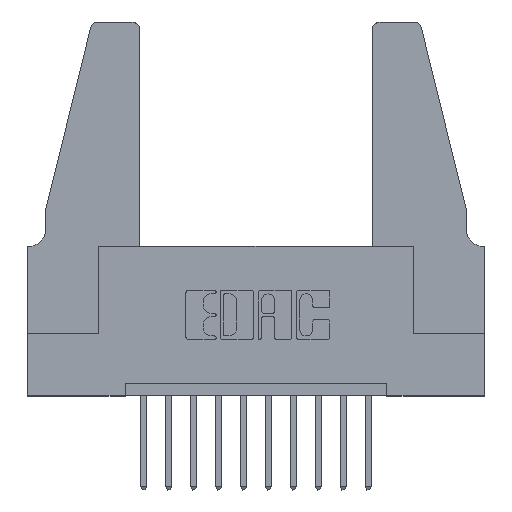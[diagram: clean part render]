
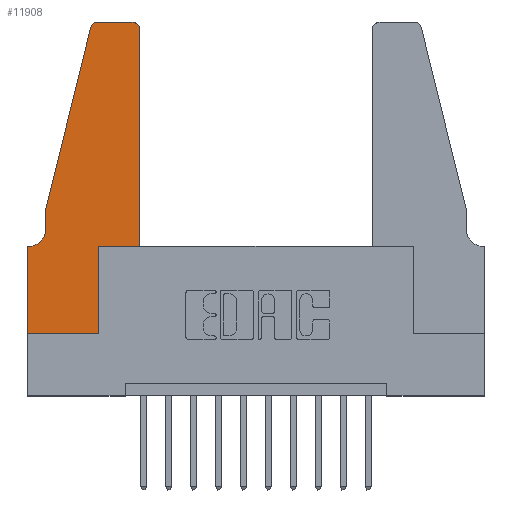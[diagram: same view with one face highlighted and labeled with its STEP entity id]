
A CAD part, top view. The second image highlights one B-rep face of the part: STEP entity #11908.
In plain terms, the highlighted planar face has unit normal (0, 0, 1).
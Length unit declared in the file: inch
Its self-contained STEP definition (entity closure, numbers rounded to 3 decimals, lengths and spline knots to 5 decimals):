
#12 = CARTESIAN_POINT ( 'NONE',  ( 0., 0., 0.37 ) ) ;
#136 = FACE_OUTER_BOUND ( 'NONE', #6134, .T. ) ;
#581 = DIRECTION ( 'NONE',  ( 1., 0., 0. ) ) ;
#858 = ORIENTED_EDGE ( 'NONE', *, *, #12434, .T. ) ;
#1010 = ORIENTED_EDGE ( 'NONE', *, *, #1583, .T. ) ;
#1086 = VECTOR ( 'NONE', #9550, 39.37008 ) ;
#1149 = ORIENTED_EDGE ( 'NONE', *, *, #5178, .T. ) ;
#1163 = EDGE_CURVE ( 'NONE', #9561, #11566, #9908, .T. ) ;
#1201 = VERTEX_POINT ( 'NONE', #7324 ) ;
#1239 = EDGE_CURVE ( 'NONE', #2091, #9561, #8863, .T. ) ;
#1376 = VERTEX_POINT ( 'NONE', #4563 ) ;
#1410 = VECTOR ( 'NONE', #8192, 39.37008 ) ;
#1583 = EDGE_CURVE ( 'NONE', #1201, #2091, #2759, .T. ) ;
#1601 = CARTESIAN_POINT ( 'NONE',  ( 0.0055, 0.35, 0.37 ) ) ;
#1678 = DIRECTION ( 'NONE',  ( 1., 0., 0. ) ) ;
#1853 = CARTESIAN_POINT ( 'NONE',  ( 0.0755, 0.5, 0.37 ) ) ;
#1860 = DIRECTION ( 'NONE',  ( -1., 0., 0. ) ) ;
#1867 = CARTESIAN_POINT ( 'NONE',  ( 0.0755, 0.35, 0.37 ) ) ;
#2091 = VERTEX_POINT ( 'NONE', #7535 ) ;
#2193 = DIRECTION ( 'NONE',  ( 0., 1., 0. ) ) ;
#2215 = DIRECTION ( 'NONE',  ( 1., 0., 0. ) ) ;
#2481 = PLANE ( 'NONE',  #9139 ) ;
#2516 = LINE ( 'NONE', #3801, #5365 ) ;
#2559 = ORIENTED_EDGE ( 'NONE', *, *, #5198, .T. ) ;
#2634 = DIRECTION ( 'NONE',  ( 0., -1., 0. ) ) ;
#2759 = LINE ( 'NONE', #3649, #7322 ) ;
#2823 = CARTESIAN_POINT ( 'NONE',  ( 0.4205, 1.22, 0.37 ) ) ;
#2989 = DIRECTION ( 'NONE',  ( -0.239, -0.971, 0. ) ) ;
#3015 = VECTOR ( 'NONE', #2634, 39.37008 ) ;
#3292 = LINE ( 'NONE', #1867, #1410 ) ;
#3458 = VECTOR ( 'NONE', #2989, 39.37008 ) ;
#3649 = CARTESIAN_POINT ( 'NONE',  ( 0.2605, 1.25, 0.37 ) ) ;
#3690 = CIRCLE ( 'NONE', #5766, 0.07 ) ;
#3783 = ORIENTED_EDGE ( 'NONE', *, *, #1163, .T. ) ;
#3801 = CARTESIAN_POINT ( 'NONE',  ( 0.0755, 0.5, 0.37 ) ) ;
#4131 = VECTOR ( 'NONE', #581, 39.37008 ) ;
#4202 = EDGE_CURVE ( 'NONE', #7536, #9682, #10486, .T. ) ;
#4563 = CARTESIAN_POINT ( 'NONE',  ( 0.2865, 0.35, 0.37 ) ) ;
#4586 = CARTESIAN_POINT ( 'NONE',  ( 0., 0.35, 0.37 ) ) ;
#4638 = ORIENTED_EDGE ( 'NONE', *, *, #11731, .T. ) ;
#4910 = VERTEX_POINT ( 'NONE', #13992 ) ;
#4999 = CARTESIAN_POINT ( 'NONE',  ( 0.0755, 0.5, 0.37 ) ) ;
#5178 = EDGE_CURVE ( 'NONE', #5572, #1201, #9120, .T. ) ;
#5193 = CARTESIAN_POINT ( 'NONE',  ( 0.0755, 0.42, 0.37 ) ) ;
#5198 = EDGE_CURVE ( 'NONE', #12837, #7536, #8088, .T. ) ;
#5216 = AXIS2_PLACEMENT_3D ( 'NONE', #2823, #9127, #1678 ) ;
#5365 = VECTOR ( 'NONE', #8186, 39.37008 ) ;
#5572 = VERTEX_POINT ( 'NONE', #6937 ) ;
#5766 = AXIS2_PLACEMENT_3D ( 'NONE', #11560, #6162, #1860 ) ;
#5963 = CARTESIAN_POINT ( 'NONE',  ( 0.4505, 0.35, 0.37 ) ) ;
#6134 = EDGE_LOOP ( 'NONE', ( #1010, #7694, #3783, #4638, #858, #13427, #2559, #9361, #13633, #8779, #10126, #1149 ) ) ;
#6162 = DIRECTION ( 'NONE',  ( 0., 0., -1. ) ) ;
#6455 = VERTEX_POINT ( 'NONE', #1601 ) ;
#6521 = CARTESIAN_POINT ( 'NONE',  ( 0.284, 1.22, 0.37 ) ) ;
#6911 = VECTOR ( 'NONE', #2193, 39.37008 ) ;
#6937 = CARTESIAN_POINT ( 'NONE',  ( 0.4505, 1.22, 0.37 ) ) ;
#7108 = EDGE_CURVE ( 'NONE', #6455, #12837, #3292, .T. ) ;
#7322 = VECTOR ( 'NONE', #12197, 39.37008 ) ;
#7324 = CARTESIAN_POINT ( 'NONE',  ( 0.4205, 1.25, 0.37 ) ) ;
#7478 = EDGE_CURVE ( 'NONE', #1376, #4910, #11598, .T. ) ;
#7503 = DIRECTION ( 'NONE',  ( 0., 0., 1. ) ) ;
#7535 = CARTESIAN_POINT ( 'NONE',  ( 0.284, 1.25, 0.37 ) ) ;
#7536 = VERTEX_POINT ( 'NONE', #12 ) ;
#7694 = ORIENTED_EDGE ( 'NONE', *, *, #1239, .T. ) ;
#8088 = LINE ( 'NONE', #9273, #3015 ) ;
#8186 = DIRECTION ( 'NONE',  ( 0., -1., 0. ) ) ;
#8192 = DIRECTION ( 'NONE',  ( -1., 0., 0. ) ) ;
#8362 = AXIS2_PLACEMENT_3D ( 'NONE', #6521, #7503, #2215 ) ;
#8404 = EDGE_CURVE ( 'NONE', #9682, #1376, #10749, .T. ) ;
#8779 = ORIENTED_EDGE ( 'NONE', *, *, #7478, .T. ) ;
#8863 = CIRCLE ( 'NONE', #8362, 0.03 ) ;
#8965 = DIRECTION ( 'NONE',  ( 0., 0., 1. ) ) ;
#9120 = CIRCLE ( 'NONE', #5216, 0.03 ) ;
#9127 = DIRECTION ( 'NONE',  ( 0., 0., 1. ) ) ;
#9139 = AXIS2_PLACEMENT_3D ( 'NONE', #4586, #8965, #12217 ) ;
#9273 = CARTESIAN_POINT ( 'NONE',  ( 0., 0., 0.37 ) ) ;
#9302 = VERTEX_POINT ( 'NONE', #5193 ) ;
#9361 = ORIENTED_EDGE ( 'NONE', *, *, #4202, .T. ) ;
#9438 = CARTESIAN_POINT ( 'NONE',  ( 0.25487, 1.22718, 0.37 ) ) ;
#9550 = DIRECTION ( 'NONE',  ( 0., 1., 0. ) ) ;
#9561 = VERTEX_POINT ( 'NONE', #9438 ) ;
#9590 = CARTESIAN_POINT ( 'NONE',  ( 0., 0., 0.37 ) ) ;
#9682 = VERTEX_POINT ( 'NONE', #11921 ) ;
#9747 = CARTESIAN_POINT ( 'NONE',  ( 0.4505, 0.35, 0.37 ) ) ;
#9908 = LINE ( 'NONE', #1853, #3458 ) ;
#10126 = ORIENTED_EDGE ( 'NONE', *, *, #11581, .T. ) ;
#10486 = LINE ( 'NONE', #9590, #10978 ) ;
#10567 = DIRECTION ( 'NONE',  ( 1., 0., 0. ) ) ;
#10749 = LINE ( 'NONE', #13789, #1086 ) ;
#10978 = VECTOR ( 'NONE', #10567, 39.37008 ) ;
#11214 = CARTESIAN_POINT ( 'NONE',  ( 0., 0.35, 0.37 ) ) ;
#11560 = CARTESIAN_POINT ( 'NONE',  ( 0.0055, 0.42, 0.37 ) ) ;
#11566 = VERTEX_POINT ( 'NONE', #4999 ) ;
#11581 = EDGE_CURVE ( 'NONE', #4910, #5572, #12675, .T. ) ;
#11598 = LINE ( 'NONE', #5963, #4131 ) ;
#11731 = EDGE_CURVE ( 'NONE', #11566, #9302, #2516, .T. ) ;
#11908 = ADVANCED_FACE ( 'NONE', ( #136 ), #2481, .T. ) ;
#11921 = CARTESIAN_POINT ( 'NONE',  ( 0.2865, 0., 0.37 ) ) ;
#12197 = DIRECTION ( 'NONE',  ( -1., 0., 0. ) ) ;
#12217 = DIRECTION ( 'NONE',  ( 1., 0., 0. ) ) ;
#12434 = EDGE_CURVE ( 'NONE', #9302, #6455, #3690, .T. ) ;
#12675 = LINE ( 'NONE', #9747, #6911 ) ;
#12837 = VERTEX_POINT ( 'NONE', #11214 ) ;
#13427 = ORIENTED_EDGE ( 'NONE', *, *, #7108, .T. ) ;
#13633 = ORIENTED_EDGE ( 'NONE', *, *, #8404, .T. ) ;
#13789 = CARTESIAN_POINT ( 'NONE',  ( 0.2865, 0.35, 0.37 ) ) ;
#13992 = CARTESIAN_POINT ( 'NONE',  ( 0.4505, 0.35, 0.37 ) ) ;
